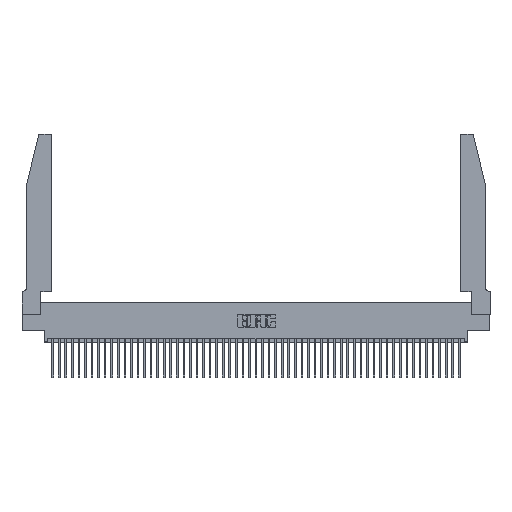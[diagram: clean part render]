
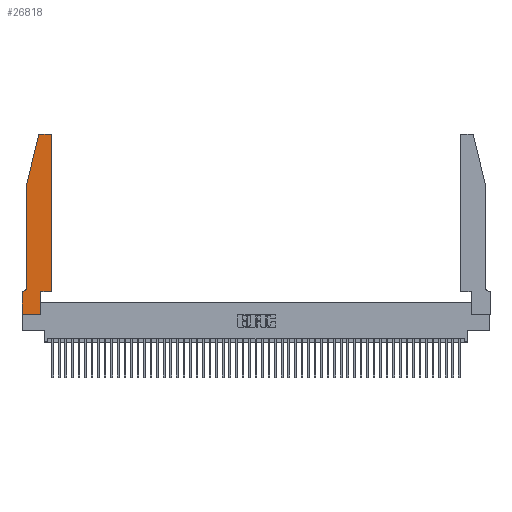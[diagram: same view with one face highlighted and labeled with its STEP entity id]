
A CAD part, top view. The second image highlights one B-rep face of the part: STEP entity #26818.
In plain terms, the highlighted planar face has unit normal (0, 0, 1).
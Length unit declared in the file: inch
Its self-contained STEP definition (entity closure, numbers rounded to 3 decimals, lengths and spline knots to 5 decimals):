
#565 = VERTEX_POINT ( 'NONE', #41576 ) ;
#1374 = VERTEX_POINT ( 'NONE', #26420 ) ;
#1593 = DIRECTION ( 'NONE',  ( -1., 0., 0. ) ) ;
#1616 = LINE ( 'NONE', #8092, #42682 ) ;
#1739 = ORIENTED_EDGE ( 'NONE', *, *, #32446, .T. ) ;
#1870 = EDGE_CURVE ( 'NONE', #1374, #46820, #46993, .T. ) ;
#2174 = LINE ( 'NONE', #7438, #43203 ) ;
#2776 = VECTOR ( 'NONE', #38555, 39.37008 ) ;
#3487 = ORIENTED_EDGE ( 'NONE', *, *, #27470, .T. ) ;
#4357 = PLANE ( 'NONE',  #7532 ) ;
#4613 = ORIENTED_EDGE ( 'NONE', *, *, #36581, .T. ) ;
#4622 = CARTESIAN_POINT ( 'NONE',  ( 0.284, 2.72, 0.37 ) ) ;
#4827 = VECTOR ( 'NONE', #23001, 39.37008 ) ;
#5252 = VECTOR ( 'NONE', #1593, 39.37008 ) ;
#5334 = ORIENTED_EDGE ( 'NONE', *, *, #21775, .T. ) ;
#5382 = CARTESIAN_POINT ( 'NONE',  ( 0.0755, 2., 0.37 ) ) ;
#5628 = AXIS2_PLACEMENT_3D ( 'NONE', #14035, #41569, #18058 ) ;
#6001 = CARTESIAN_POINT ( 'NONE',  ( 0.2865, 0.35, 0.37 ) ) ;
#6662 = LINE ( 'NONE', #15000, #2776 ) ;
#7438 = CARTESIAN_POINT ( 'NONE',  ( 0., 0., 0.37 ) ) ;
#7532 = AXIS2_PLACEMENT_3D ( 'NONE', #32069, #12567, #40073 ) ;
#8092 = CARTESIAN_POINT ( 'NONE',  ( 0.0755, 2., 0.37 ) ) ;
#8754 = DIRECTION ( 'NONE',  ( 1., 0., 0. ) ) ;
#9144 = VECTOR ( 'NONE', #15453, 39.37008 ) ;
#9647 = VERTEX_POINT ( 'NONE', #28577 ) ;
#11453 = EDGE_CURVE ( 'NONE', #18185, #14630, #13060, .T. ) ;
#11470 = VERTEX_POINT ( 'NONE', #44964 ) ;
#11608 = CARTESIAN_POINT ( 'NONE',  ( 0.4205, 2.72, 0.37 ) ) ;
#11885 = CARTESIAN_POINT ( 'NONE',  ( 0.284, 2.75, 0.37 ) ) ;
#12159 = DIRECTION ( 'NONE',  ( -0.239, -0.971, 0. ) ) ;
#12567 = DIRECTION ( 'NONE',  ( 0., 0., 1. ) ) ;
#12582 = EDGE_CURVE ( 'NONE', #9647, #1374, #35219, .T. ) ;
#13060 = LINE ( 'NONE', #33135, #22363 ) ;
#13462 = DIRECTION ( 'NONE',  ( 1., 0., 0. ) ) ;
#13680 = CARTESIAN_POINT ( 'NONE',  ( 0., 0.35, 0.37 ) ) ;
#14035 = CARTESIAN_POINT ( 'NONE',  ( 0.0055, 0.42, 0.37 ) ) ;
#14630 = VERTEX_POINT ( 'NONE', #39017 ) ;
#15000 = CARTESIAN_POINT ( 'NONE',  ( 0.2865, 0.35, 0.37 ) ) ;
#15453 = DIRECTION ( 'NONE',  ( 0., -1., 0. ) ) ;
#15611 = VECTOR ( 'NONE', #24624, 39.37008 ) ;
#15627 = DIRECTION ( 'NONE',  ( 1., 0., 0. ) ) ;
#16737 = CARTESIAN_POINT ( 'NONE',  ( 0.0055, 0.35, 0.37 ) ) ;
#17623 = ORIENTED_EDGE ( 'NONE', *, *, #27350, .T. ) ;
#18058 = DIRECTION ( 'NONE',  ( -1., 0., 0. ) ) ;
#18185 = VERTEX_POINT ( 'NONE', #6001 ) ;
#18455 = CARTESIAN_POINT ( 'NONE',  ( 0., 0., 0.37 ) ) ;
#18559 = VERTEX_POINT ( 'NONE', #28093 ) ;
#20713 = EDGE_CURVE ( 'NONE', #40214, #18185, #6662, .T. ) ;
#20847 = AXIS2_PLACEMENT_3D ( 'NONE', #11608, #39173, #15627 ) ;
#21775 = EDGE_CURVE ( 'NONE', #565, #26859, #49489, .T. ) ;
#21967 = ORIENTED_EDGE ( 'NONE', *, *, #12582, .T. ) ;
#22363 = VECTOR ( 'NONE', #13462, 39.37008 ) ;
#23001 = DIRECTION ( 'NONE',  ( -1., 0., 0. ) ) ;
#23892 = EDGE_CURVE ( 'NONE', #26859, #42573, #34483, .T. ) ;
#24624 = DIRECTION ( 'NONE',  ( 0., -1., 0. ) ) ;
#25691 = CARTESIAN_POINT ( 'NONE',  ( 0.0755, 0.35, 0.37 ) ) ;
#26392 = DIRECTION ( 'NONE',  ( 0., 1., 0. ) ) ;
#26420 = CARTESIAN_POINT ( 'NONE',  ( 0.4205, 2.75, 0.37 ) ) ;
#26818 = ADVANCED_FACE ( 'NONE', ( #46458 ), #4357, .T. ) ;
#26859 = VERTEX_POINT ( 'NONE', #16737 ) ;
#27350 = EDGE_CURVE ( 'NONE', #18559, #11470, #1616, .T. ) ;
#27470 = EDGE_CURVE ( 'NONE', #11470, #565, #36548, .T. ) ;
#27697 = CARTESIAN_POINT ( 'NONE',  ( 0.2865, 0., 0.37 ) ) ;
#28080 = CIRCLE ( 'NONE', #37095, 0.03 ) ;
#28093 = CARTESIAN_POINT ( 'NONE',  ( 0.25487, 2.72718, 0.37 ) ) ;
#28577 = CARTESIAN_POINT ( 'NONE',  ( 0.4505, 2.72, 0.37 ) ) ;
#28909 = EDGE_CURVE ( 'NONE', #46820, #18559, #28080, .T. ) ;
#29527 = ORIENTED_EDGE ( 'NONE', *, *, #11453, .T. ) ;
#30271 = ORIENTED_EDGE ( 'NONE', *, *, #40109, .T. ) ;
#31521 = ORIENTED_EDGE ( 'NONE', *, *, #28909, .T. ) ;
#32069 = CARTESIAN_POINT ( 'NONE',  ( 0., 0.35, 0.37 ) ) ;
#32446 = EDGE_CURVE ( 'NONE', #14630, #9647, #47388, .T. ) ;
#32508 = DIRECTION ( 'NONE',  ( 0., 0., 1. ) ) ;
#33135 = CARTESIAN_POINT ( 'NONE',  ( 0.4505, 0.35, 0.37 ) ) ;
#33879 = ORIENTED_EDGE ( 'NONE', *, *, #23892, .T. ) ;
#34483 = LINE ( 'NONE', #25691, #5252 ) ;
#35081 = CARTESIAN_POINT ( 'NONE',  ( 0., 0., 0.37 ) ) ;
#35219 = CIRCLE ( 'NONE', #20847, 0.03 ) ;
#36548 = LINE ( 'NONE', #5382, #15611 ) ;
#36581 = EDGE_CURVE ( 'NONE', #51513, #40214, #2174, .T. ) ;
#36932 = VECTOR ( 'NONE', #26392, 39.37008 ) ;
#37095 = AXIS2_PLACEMENT_3D ( 'NONE', #4622, #32508, #8754 ) ;
#38042 = CARTESIAN_POINT ( 'NONE',  ( 0.4505, 0.35, 0.37 ) ) ;
#38555 = DIRECTION ( 'NONE',  ( 0., 1., 0. ) ) ;
#39017 = CARTESIAN_POINT ( 'NONE',  ( 0.4505, 0.35, 0.37 ) ) ;
#39173 = DIRECTION ( 'NONE',  ( 0., 0., 1. ) ) ;
#40073 = DIRECTION ( 'NONE',  ( 1., 0., 0. ) ) ;
#40109 = EDGE_CURVE ( 'NONE', #42573, #51513, #43115, .T. ) ;
#40214 = VERTEX_POINT ( 'NONE', #27697 ) ;
#41104 = ORIENTED_EDGE ( 'NONE', *, *, #20713, .T. ) ;
#41569 = DIRECTION ( 'NONE',  ( 0., 0., -1. ) ) ;
#41576 = CARTESIAN_POINT ( 'NONE',  ( 0.0755, 0.42, 0.37 ) ) ;
#42573 = VERTEX_POINT ( 'NONE', #13680 ) ;
#42682 = VECTOR ( 'NONE', #12159, 39.37008 ) ;
#43115 = LINE ( 'NONE', #35081, #9144 ) ;
#43203 = VECTOR ( 'NONE', #47015, 39.37008 ) ;
#44964 = CARTESIAN_POINT ( 'NONE',  ( 0.0755, 2., 0.37 ) ) ;
#45120 = EDGE_LOOP ( 'NONE', ( #46750, #31521, #17623, #3487, #5334, #33879, #30271, #4613, #41104, #29527, #1739, #21967 ) ) ;
#46458 = FACE_OUTER_BOUND ( 'NONE', #45120, .T. ) ;
#46750 = ORIENTED_EDGE ( 'NONE', *, *, #1870, .T. ) ;
#46820 = VERTEX_POINT ( 'NONE', #11885 ) ;
#46993 = LINE ( 'NONE', #50511, #4827 ) ;
#47015 = DIRECTION ( 'NONE',  ( 1., 0., 0. ) ) ;
#47388 = LINE ( 'NONE', #38042, #36932 ) ;
#49489 = CIRCLE ( 'NONE', #5628, 0.07 ) ;
#50511 = CARTESIAN_POINT ( 'NONE',  ( 0.2605, 2.75, 0.37 ) ) ;
#51513 = VERTEX_POINT ( 'NONE', #18455 ) ;
